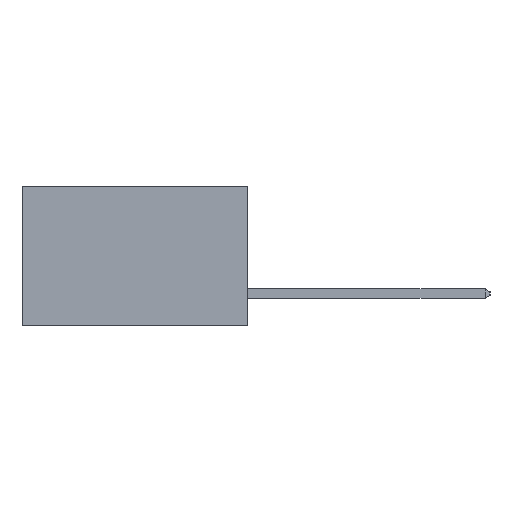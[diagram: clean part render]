
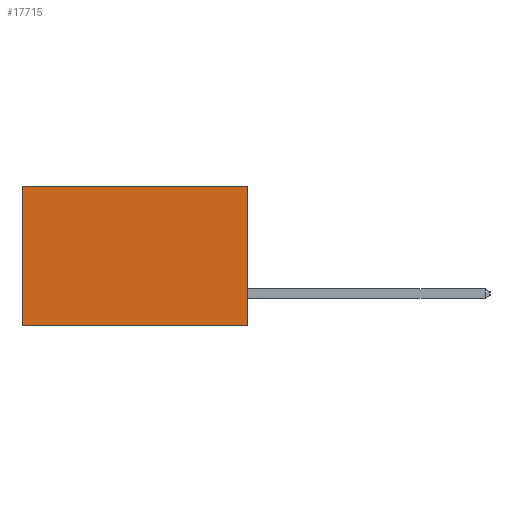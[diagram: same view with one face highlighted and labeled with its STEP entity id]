
A CAD part, left-side view. The second image highlights one B-rep face of the part: STEP entity #17715.
In plain terms, the highlighted planar face has unit normal (-1, 0, 0).
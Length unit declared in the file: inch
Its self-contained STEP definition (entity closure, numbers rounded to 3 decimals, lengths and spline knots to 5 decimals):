
#384 = FACE_OUTER_BOUND ( 'NONE', #17058, .T. ) ;
#738 = VECTOR ( 'NONE', #3113, 39.37008 ) ;
#1715 = DIRECTION ( 'NONE',  ( 0., 0., -1. ) ) ;
#3113 = DIRECTION ( 'NONE',  ( 0., 1., 0. ) ) ;
#3969 = VERTEX_POINT ( 'NONE', #11121 ) ;
#3978 = ORIENTED_EDGE ( 'NONE', *, *, #13042, .T. ) ;
#4105 = EDGE_CURVE ( 'NONE', #10819, #7338, #12094, .T. ) ;
#5985 = CARTESIAN_POINT ( 'NONE',  ( 0.298, 0., 0. ) ) ;
#6048 = DIRECTION ( 'NONE',  ( 0., 1., 0. ) ) ;
#6094 = VECTOR ( 'NONE', #17722, 39.37008 ) ;
#6367 = CARTESIAN_POINT ( 'NONE',  ( 0.298, 0., -0.37 ) ) ;
#6690 = CARTESIAN_POINT ( 'NONE',  ( 0.298, 0., 0. ) ) ;
#6700 = CARTESIAN_POINT ( 'NONE',  ( 0.298, 0.6, 0. ) ) ;
#7338 = VERTEX_POINT ( 'NONE', #12452 ) ;
#7546 = VECTOR ( 'NONE', #1715, 39.37008 ) ;
#7617 = AXIS2_PLACEMENT_3D ( 'NONE', #6690, #16352, #8107 ) ;
#7862 = LINE ( 'NONE', #14307, #738 ) ;
#8107 = DIRECTION ( 'NONE',  ( 0., 0., -1. ) ) ;
#8697 = ORIENTED_EDGE ( 'NONE', *, *, #4105, .F. ) ;
#8775 = CARTESIAN_POINT ( 'NONE',  ( 0.298, 0., -0.37 ) ) ;
#9849 = LINE ( 'NONE', #6700, #6094 ) ;
#10070 = ORIENTED_EDGE ( 'NONE', *, *, #12723, .T. ) ;
#10819 = VERTEX_POINT ( 'NONE', #6367 ) ;
#10863 = LINE ( 'NONE', #5985, #7546 ) ;
#11121 = CARTESIAN_POINT ( 'NONE',  ( 0.298, 0.6, 0. ) ) ;
#11432 = VERTEX_POINT ( 'NONE', #14825 ) ;
#12094 = LINE ( 'NONE', #8775, #15266 ) ;
#12452 = CARTESIAN_POINT ( 'NONE',  ( 0.298, 0.6, -0.37 ) ) ;
#12723 = EDGE_CURVE ( 'NONE', #3969, #7338, #9849, .T. ) ;
#13042 = EDGE_CURVE ( 'NONE', #11432, #3969, #7862, .T. ) ;
#13626 = PLANE ( 'NONE',  #7617 ) ;
#14307 = CARTESIAN_POINT ( 'NONE',  ( 0.298, 0., 0. ) ) ;
#14825 = CARTESIAN_POINT ( 'NONE',  ( 0.298, 0., 0. ) ) ;
#15266 = VECTOR ( 'NONE', #6048, 39.37008 ) ;
#15351 = EDGE_CURVE ( 'NONE', #11432, #10819, #10863, .T. ) ;
#16352 = DIRECTION ( 'NONE',  ( 1., 0., 0. ) ) ;
#16462 = ORIENTED_EDGE ( 'NONE', *, *, #15351, .F. ) ;
#17058 = EDGE_LOOP ( 'NONE', ( #10070, #8697, #16462, #3978 ) ) ;
#17715 = ADVANCED_FACE ( 'NONE', ( #384 ), #13626, .F. ) ;
#17722 = DIRECTION ( 'NONE',  ( 0., 0., -1. ) ) ;
